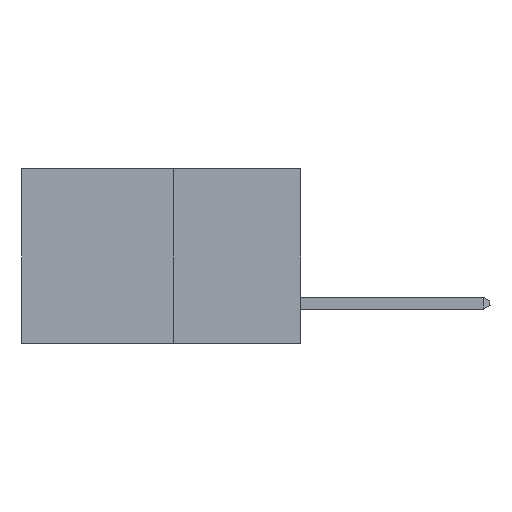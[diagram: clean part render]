
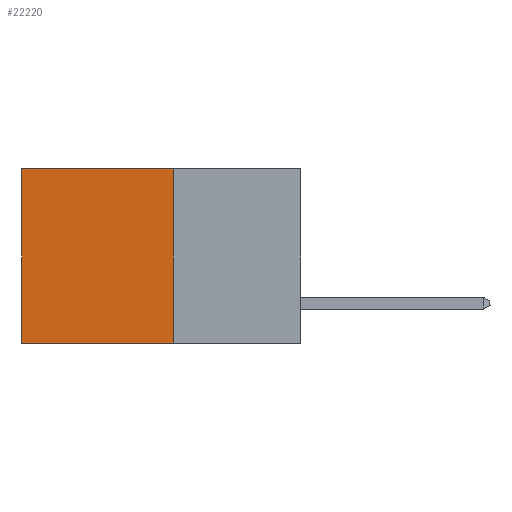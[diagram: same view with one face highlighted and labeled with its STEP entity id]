
A CAD part, left-side view. The second image highlights one B-rep face of the part: STEP entity #22220.
In plain terms, the highlighted planar face has unit normal (-1, 0, 0).
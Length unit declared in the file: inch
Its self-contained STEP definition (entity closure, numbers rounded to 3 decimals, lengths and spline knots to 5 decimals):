
#160 = LINE ( 'NONE', #12844, #30846 ) ;
#729 = DIRECTION ( 'NONE',  ( 0., 1., 0. ) ) ;
#3605 = DIRECTION ( 'NONE',  ( 0., 0., -1. ) ) ;
#4153 = CARTESIAN_POINT ( 'NONE',  ( 0.277, 0.27, -0.37 ) ) ;
#4175 = VECTOR ( 'NONE', #3605, 39.37008 ) ;
#4398 = EDGE_CURVE ( 'NONE', #22759, #28305, #22648, .T. ) ;
#4671 = LINE ( 'NONE', #4153, #16771 ) ;
#5656 = VECTOR ( 'NONE', #27842, 39.37008 ) ;
#6653 = DIRECTION ( 'NONE',  ( 0., 1., 0. ) ) ;
#7003 = CARTESIAN_POINT ( 'NONE',  ( 0.277, 0.59, 0. ) ) ;
#9460 = PLANE ( 'NONE',  #25666 ) ;
#10090 = ORIENTED_EDGE ( 'NONE', *, *, #21443, .F. ) ;
#10793 = VERTEX_POINT ( 'NONE', #17971 ) ;
#11886 = DIRECTION ( 'NONE',  ( 0., 0., -1. ) ) ;
#12418 = ORIENTED_EDGE ( 'NONE', *, *, #29773, .F. ) ;
#12844 = CARTESIAN_POINT ( 'NONE',  ( 0.277, 0.27, 0. ) ) ;
#14142 = VERTEX_POINT ( 'NONE', #16547 ) ;
#14736 = EDGE_LOOP ( 'NONE', ( #16175, #10090, #12418, #30356 ) ) ;
#16175 = ORIENTED_EDGE ( 'NONE', *, *, #4398, .T. ) ;
#16547 = CARTESIAN_POINT ( 'NONE',  ( 0.277, 0.27, -0.37 ) ) ;
#16609 = CARTESIAN_POINT ( 'NONE',  ( 0.277, 0.27, -0.37 ) ) ;
#16771 = VECTOR ( 'NONE', #6653, 39.37008 ) ;
#17460 = CARTESIAN_POINT ( 'NONE',  ( 0.277, 0.59, -0.37 ) ) ;
#17830 = LINE ( 'NONE', #20689, #4175 ) ;
#17971 = CARTESIAN_POINT ( 'NONE',  ( 0.277, 0.27, 0. ) ) ;
#20175 = CARTESIAN_POINT ( 'NONE',  ( 0.277, 0.59, -0.37 ) ) ;
#20689 = CARTESIAN_POINT ( 'NONE',  ( 0.277, 0.27, -0.37 ) ) ;
#21443 = EDGE_CURVE ( 'NONE', #14142, #28305, #4671, .T. ) ;
#22220 = ADVANCED_FACE ( 'NONE', ( #25442 ), #9460, .F. ) ;
#22648 = LINE ( 'NONE', #20175, #5656 ) ;
#22759 = VERTEX_POINT ( 'NONE', #7003 ) ;
#23696 = EDGE_CURVE ( 'NONE', #10793, #22759, #160, .T. ) ;
#25442 = FACE_OUTER_BOUND ( 'NONE', #14736, .T. ) ;
#25666 = AXIS2_PLACEMENT_3D ( 'NONE', #16609, #26374, #11886 ) ;
#26374 = DIRECTION ( 'NONE',  ( 1., 0., 0. ) ) ;
#27842 = DIRECTION ( 'NONE',  ( 0., 0., -1. ) ) ;
#28305 = VERTEX_POINT ( 'NONE', #17460 ) ;
#29773 = EDGE_CURVE ( 'NONE', #10793, #14142, #17830, .T. ) ;
#30356 = ORIENTED_EDGE ( 'NONE', *, *, #23696, .T. ) ;
#30846 = VECTOR ( 'NONE', #729, 39.37008 ) ;
